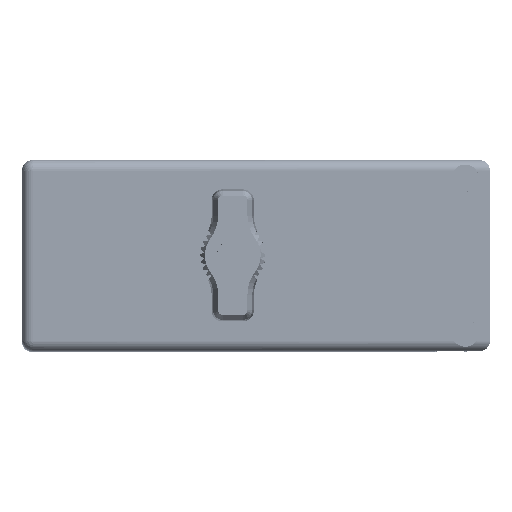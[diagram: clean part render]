
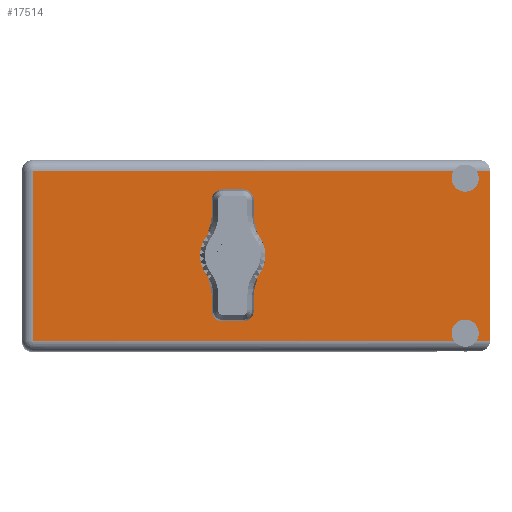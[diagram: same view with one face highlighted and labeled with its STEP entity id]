
A CAD part, top view. The second image highlights one B-rep face of the part: STEP entity #17514.
In plain terms, the highlighted face is planar.
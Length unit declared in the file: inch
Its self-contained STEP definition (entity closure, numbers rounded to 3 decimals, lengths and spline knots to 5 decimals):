
#292 = LINE ( 'NONE', #27558, #33736 ) ;
#1461 = DIRECTION ( 'NONE',  ( 0., 1., 0. ) ) ;
#1880 = CARTESIAN_POINT ( 'NONE',  ( 1.57281, 1.675, -0.547 ) ) ;
#2046 = VECTOR ( 'NONE', #73595, 39.37008 ) ;
#3061 = PLANE ( 'NONE',  #61446 ) ;
#3805 = LINE ( 'NONE', #18462, #72858 ) ;
#4271 = EDGE_LOOP ( 'NONE', ( #65507, #30880 ) ) ;
#5384 = VERTEX_POINT ( 'NONE', #83252 ) ;
#6253 = ORIENTED_EDGE ( 'NONE', *, *, #8338, .F. ) ;
#6331 = LINE ( 'NONE', #79065, #19909 ) ;
#8338 = EDGE_CURVE ( 'NONE', #51728, #73756, #63691, .T. ) ;
#9482 = ORIENTED_EDGE ( 'NONE', *, *, #29921, .T. ) ;
#10717 = CIRCLE ( 'NONE', #42857, 0.125 ) ;
#12682 = FACE_BOUND ( 'NONE', #4271, .T. ) ;
#13299 = DIRECTION ( 'NONE',  ( 0., 0., 1. ) ) ;
#14631 = CARTESIAN_POINT ( 'NONE',  ( 0., 1.675, 0. ) ) ;
#14645 = CIRCLE ( 'NONE', #58904, 0.0875 ) ;
#16143 = EDGE_CURVE ( 'NONE', #58519, #23137, #10717, .T. ) ;
#16238 = CARTESIAN_POINT ( 'NONE',  ( 1.499, 1.675, -0.5 ) ) ;
#17446 = ORIENTED_EDGE ( 'NONE', *, *, #55057, .T. ) ;
#17514 = ADVANCED_FACE ( 'NONE', ( #12682, #46010 ), #3061, .T. ) ;
#18462 = CARTESIAN_POINT ( 'NONE',  ( 1.659, 1.675, 0.547 ) ) ;
#19909 = VECTOR ( 'NONE', #60057, 39.37008 ) ;
#20314 = ORIENTED_EDGE ( 'NONE', *, *, #52880, .T. ) ;
#21232 = CARTESIAN_POINT ( 'NONE',  ( 1.659, 1.675, -0.547 ) ) ;
#21809 = VERTEX_POINT ( 'NONE', #73983 ) ;
#21960 = DIRECTION ( 'NONE',  ( 0., 1., 0. ) ) ;
#22360 = CIRCLE ( 'NONE', #24946, 0.0875 ) ;
#23137 = VERTEX_POINT ( 'NONE', #61819 ) ;
#24946 = AXIS2_PLACEMENT_3D ( 'NONE', #16238, #69485, #62176 ) ;
#25722 = EDGE_CURVE ( 'NONE', #84349, #44016, #22360, .T. ) ;
#26563 = CARTESIAN_POINT ( 'NONE',  ( -1.289, 1.675, -0.617 ) ) ;
#27558 = CARTESIAN_POINT ( 'NONE',  ( 1.659, 1.675, 0.547 ) ) ;
#28350 = VECTOR ( 'NONE', #64734, 39.37008 ) ;
#28675 = DIRECTION ( 'NONE',  ( 0., 0., 1. ) ) ;
#29921 = EDGE_CURVE ( 'NONE', #5384, #21809, #292, .T. ) ;
#30543 = EDGE_CURVE ( 'NONE', #23137, #58519, #83838, .T. ) ;
#30789 = ORIENTED_EDGE ( 'NONE', *, *, #69913, .T. ) ;
#30880 = ORIENTED_EDGE ( 'NONE', *, *, #30543, .F. ) ;
#30907 = ORIENTED_EDGE ( 'NONE', *, *, #72976, .F. ) ;
#32004 = CARTESIAN_POINT ( 'NONE',  ( 1.499, 1.675, 0.5 ) ) ;
#32863 = CARTESIAN_POINT ( 'NONE',  ( 1.42519, 1.675, -0.547 ) ) ;
#33736 = VECTOR ( 'NONE', #81654, 39.37008 ) ;
#35207 = CARTESIAN_POINT ( 'NONE',  ( -1.289, 1.675, 0.547 ) ) ;
#35599 = VECTOR ( 'NONE', #38676, 39.37008 ) ;
#35806 = VERTEX_POINT ( 'NONE', #21232 ) ;
#38204 = DIRECTION ( 'NONE',  ( 0., 1., 0. ) ) ;
#38676 = DIRECTION ( 'NONE',  ( -1., 0., 0. ) ) ;
#39885 = LINE ( 'NONE', #64150, #28350 ) ;
#42006 = DIRECTION ( 'NONE',  ( 0., 1., 0. ) ) ;
#42015 = DIRECTION ( 'NONE',  ( 0., 0., 1. ) ) ;
#42812 = LINE ( 'NONE', #26563, #2046 ) ;
#42857 = AXIS2_PLACEMENT_3D ( 'NONE', #14631, #1461, #68433 ) ;
#43912 = CARTESIAN_POINT ( 'NONE',  ( 1.499, 1.675, -0.4125 ) ) ;
#44016 = VERTEX_POINT ( 'NONE', #1880 ) ;
#45157 = CARTESIAN_POINT ( 'NONE',  ( -1.359, 1.675, -0.547 ) ) ;
#46010 = FACE_OUTER_BOUND ( 'NONE', #75868, .T. ) ;
#47178 = LINE ( 'NONE', #45157, #35599 ) ;
#47226 = CARTESIAN_POINT ( 'NONE',  ( 1.499, 1.675, 0.4125 ) ) ;
#48007 = CARTESIAN_POINT ( 'NONE',  ( 1.499, 1.675, -0.5 ) ) ;
#49850 = CARTESIAN_POINT ( 'NONE',  ( -1.359, 1.675, -0.617 ) ) ;
#51274 = AXIS2_PLACEMENT_3D ( 'NONE', #74735, #54563, #42015 ) ;
#51728 = VERTEX_POINT ( 'NONE', #47226 ) ;
#51894 = VERTEX_POINT ( 'NONE', #69871 ) ;
#52880 = EDGE_CURVE ( 'NONE', #55901, #73756, #3805, .T. ) ;
#54563 = DIRECTION ( 'NONE',  ( 0., 1., 0. ) ) ;
#55057 = EDGE_CURVE ( 'NONE', #51894, #55901, #42812, .T. ) ;
#55901 = VERTEX_POINT ( 'NONE', #35207 ) ;
#56556 = DIRECTION ( 'NONE',  ( -1., 0., 0. ) ) ;
#56722 = ORIENTED_EDGE ( 'NONE', *, *, #61050, .F. ) ;
#58519 = VERTEX_POINT ( 'NONE', #63972 ) ;
#58904 = AXIS2_PLACEMENT_3D ( 'NONE', #32004, #38204, #65994 ) ;
#60057 = DIRECTION ( 'NONE',  ( -1., 0., 0. ) ) ;
#61050 = EDGE_CURVE ( 'NONE', #5384, #51728, #14645, .T. ) ;
#61446 = AXIS2_PLACEMENT_3D ( 'NONE', #49850, #42006, #56556 ) ;
#61819 = CARTESIAN_POINT ( 'NONE',  ( 0., 1.675, -0.125 ) ) ;
#62176 = DIRECTION ( 'NONE',  ( 0., 0., 1. ) ) ;
#63691 = CIRCLE ( 'NONE', #51274, 0.0875 ) ;
#63972 = CARTESIAN_POINT ( 'NONE',  ( 0., 1.675, 0.125 ) ) ;
#64150 = CARTESIAN_POINT ( 'NONE',  ( 1.659, 1.675, 0.617 ) ) ;
#64734 = DIRECTION ( 'NONE',  ( 0., 0., 1. ) ) ;
#65507 = ORIENTED_EDGE ( 'NONE', *, *, #16143, .F. ) ;
#65994 = DIRECTION ( 'NONE',  ( 0., 0., 1. ) ) ;
#66747 = DIRECTION ( 'NONE',  ( 0., 1., 0. ) ) ;
#67624 = CARTESIAN_POINT ( 'NONE',  ( 0., 1.675, 0. ) ) ;
#67833 = EDGE_CURVE ( 'NONE', #35806, #21809, #39885, .T. ) ;
#68433 = DIRECTION ( 'NONE',  ( 0., 0., 1. ) ) ;
#69485 = DIRECTION ( 'NONE',  ( 0., 1., 0. ) ) ;
#69709 = EDGE_CURVE ( 'NONE', #77933, #51894, #47178, .T. ) ;
#69871 = CARTESIAN_POINT ( 'NONE',  ( -1.289, 1.675, -0.547 ) ) ;
#69913 = EDGE_CURVE ( 'NONE', #35806, #44016, #6331, .T. ) ;
#71173 = AXIS2_PLACEMENT_3D ( 'NONE', #67624, #66747, #13299 ) ;
#71985 = DIRECTION ( 'NONE',  ( 1., 0., 0. ) ) ;
#72858 = VECTOR ( 'NONE', #71985, 39.37008 ) ;
#72976 = EDGE_CURVE ( 'NONE', #77933, #84349, #86228, .T. ) ;
#73551 = ORIENTED_EDGE ( 'NONE', *, *, #67833, .F. ) ;
#73595 = DIRECTION ( 'NONE',  ( 0., 0., 1. ) ) ;
#73756 = VERTEX_POINT ( 'NONE', #84350 ) ;
#73983 = CARTESIAN_POINT ( 'NONE',  ( 1.659, 1.675, 0.547 ) ) ;
#74735 = CARTESIAN_POINT ( 'NONE',  ( 1.499, 1.675, 0.5 ) ) ;
#75534 = ORIENTED_EDGE ( 'NONE', *, *, #69709, .T. ) ;
#75868 = EDGE_LOOP ( 'NONE', ( #20314, #6253, #56722, #9482, #73551, #30789, #76805, #30907, #75534, #17446 ) ) ;
#76805 = ORIENTED_EDGE ( 'NONE', *, *, #25722, .F. ) ;
#77933 = VERTEX_POINT ( 'NONE', #32863 ) ;
#79065 = CARTESIAN_POINT ( 'NONE',  ( -1.359, 1.675, -0.547 ) ) ;
#81654 = DIRECTION ( 'NONE',  ( 1., 0., 0. ) ) ;
#82953 = AXIS2_PLACEMENT_3D ( 'NONE', #48007, #21960, #28675 ) ;
#83252 = CARTESIAN_POINT ( 'NONE',  ( 1.57281, 1.675, 0.547 ) ) ;
#83838 = CIRCLE ( 'NONE', #71173, 0.125 ) ;
#84349 = VERTEX_POINT ( 'NONE', #43912 ) ;
#84350 = CARTESIAN_POINT ( 'NONE',  ( 1.42519, 1.675, 0.547 ) ) ;
#86228 = CIRCLE ( 'NONE', #82953, 0.0875 ) ;
